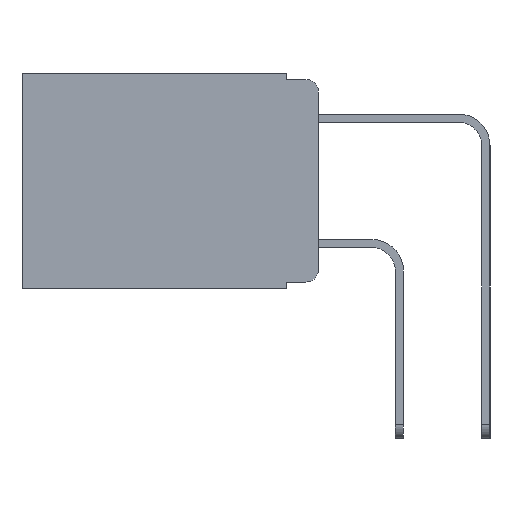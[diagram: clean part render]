
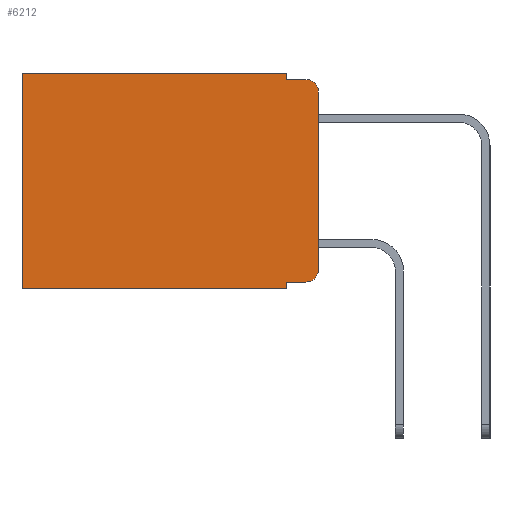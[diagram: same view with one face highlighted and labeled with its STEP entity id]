
A CAD part, left-side view. The second image highlights one B-rep face of the part: STEP entity #6212.
In plain terms, the highlighted planar face has unit normal (-1, 0, 0).
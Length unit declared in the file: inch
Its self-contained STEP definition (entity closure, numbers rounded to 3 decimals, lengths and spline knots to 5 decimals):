
#536 = LINE ( 'NONE', #10574, #8673 ) ;
#865 = CARTESIAN_POINT ( 'NONE',  ( 0.298, 0.473, 0. ) ) ;
#885 = ORIENTED_EDGE ( 'NONE', *, *, #20731, .F. ) ;
#1170 = ORIENTED_EDGE ( 'NONE', *, *, #5520, .T. ) ;
#1482 = VERTEX_POINT ( 'NONE', #12578 ) ;
#1558 = CIRCLE ( 'NONE', #4630, 0.02 ) ;
#2705 = EDGE_CURVE ( 'NONE', #1482, #16209, #9007, .T. ) ;
#2719 = ORIENTED_EDGE ( 'NONE', *, *, #12530, .T. ) ;
#3140 = CARTESIAN_POINT ( 'NONE',  ( 0.298, 0., -0.03 ) ) ;
#3523 = CARTESIAN_POINT ( 'NONE',  ( 0.298, 0., 0. ) ) ;
#3620 = CARTESIAN_POINT ( 'NONE',  ( 0.298, 0.02, -0.333 ) ) ;
#4028 = VECTOR ( 'NONE', #13603, 39.37008 ) ;
#4142 = VERTEX_POINT ( 'NONE', #865 ) ;
#4434 = CARTESIAN_POINT ( 'NONE',  ( 0.298, 0.02, -0.03 ) ) ;
#4630 = AXIS2_PLACEMENT_3D ( 'NONE', #4434, #22246, #15736 ) ;
#5473 = CARTESIAN_POINT ( 'NONE',  ( 0.298, 0., -0.313 ) ) ;
#5520 = EDGE_CURVE ( 'NONE', #17731, #4142, #17929, .T. ) ;
#5743 = CARTESIAN_POINT ( 'NONE',  ( 0.298, 0.051, -0.01 ) ) ;
#6090 = DIRECTION ( 'NONE',  ( 0., 0., -1. ) ) ;
#6212 = ADVANCED_FACE ( 'NONE', ( #18180 ), #18101, .F. ) ;
#6329 = DIRECTION ( 'NONE',  ( 0., 0., -1. ) ) ;
#6788 = VERTEX_POINT ( 'NONE', #5473 ) ;
#6921 = LINE ( 'NONE', #17741, #20232 ) ;
#7203 = VERTEX_POINT ( 'NONE', #14948 ) ;
#7598 = ORIENTED_EDGE ( 'NONE', *, *, #2705, .T. ) ;
#7611 = DIRECTION ( 'NONE',  ( 0., -1., 0. ) ) ;
#7871 = VERTEX_POINT ( 'NONE', #9380 ) ;
#8108 = CARTESIAN_POINT ( 'NONE',  ( 0.298, 0.473, -0.343 ) ) ;
#8127 = EDGE_CURVE ( 'NONE', #10082, #6788, #9394, .T. ) ;
#8179 = VECTOR ( 'NONE', #6090, 39.37008 ) ;
#8326 = ORIENTED_EDGE ( 'NONE', *, *, #8127, .F. ) ;
#8637 = VECTOR ( 'NONE', #7611, 39.37008 ) ;
#8649 = EDGE_CURVE ( 'NONE', #10082, #7871, #1558, .T. ) ;
#8673 = VECTOR ( 'NONE', #12392, 39.37008 ) ;
#8676 = EDGE_LOOP ( 'NONE', ( #8326, #15690, #21922, #22756, #1170, #11644, #885, #20040, #7598, #2719 ) ) ;
#8715 = DIRECTION ( 'NONE',  ( 0., 1., 0. ) ) ;
#9007 = LINE ( 'NONE', #18710, #22789 ) ;
#9380 = CARTESIAN_POINT ( 'NONE',  ( 0.298, 0.02, -0.01 ) ) ;
#9394 = LINE ( 'NONE', #3523, #13636 ) ;
#9458 = EDGE_CURVE ( 'NONE', #1482, #7203, #13002, .T. ) ;
#10082 = VERTEX_POINT ( 'NONE', #3140 ) ;
#10359 = VERTEX_POINT ( 'NONE', #11546 ) ;
#10502 = CARTESIAN_POINT ( 'NONE',  ( 0.298, 0.02, -0.313 ) ) ;
#10574 = CARTESIAN_POINT ( 'NONE',  ( 0.298, 0.473, 0. ) ) ;
#11546 = CARTESIAN_POINT ( 'NONE',  ( 0.298, 0.051, -0.01 ) ) ;
#11644 = ORIENTED_EDGE ( 'NONE', *, *, #20216, .T. ) ;
#11695 = CARTESIAN_POINT ( 'NONE',  ( 0.298, 0.051, 0. ) ) ;
#12268 = VECTOR ( 'NONE', #6329, 39.37008 ) ;
#12311 = DIRECTION ( 'NONE',  ( 0., 0., -1. ) ) ;
#12392 = DIRECTION ( 'NONE',  ( 0., 0., -1. ) ) ;
#12530 = EDGE_CURVE ( 'NONE', #16209, #6788, #13969, .T. ) ;
#12578 = CARTESIAN_POINT ( 'NONE',  ( 0.298, 0.051, -0.333 ) ) ;
#12847 = CARTESIAN_POINT ( 'NONE',  ( 0.298, 0., 0. ) ) ;
#13002 = LINE ( 'NONE', #22092, #8179 ) ;
#13455 = LINE ( 'NONE', #5743, #8637 ) ;
#13603 = DIRECTION ( 'NONE',  ( 0., 1., 0. ) ) ;
#13636 = VECTOR ( 'NONE', #17037, 39.37008 ) ;
#13969 = CIRCLE ( 'NONE', #21072, 0.02 ) ;
#14627 = EDGE_CURVE ( 'NONE', #10359, #7871, #13455, .T. ) ;
#14948 = CARTESIAN_POINT ( 'NONE',  ( 0.298, 0.051, -0.343 ) ) ;
#15690 = ORIENTED_EDGE ( 'NONE', *, *, #8649, .T. ) ;
#15736 = DIRECTION ( 'NONE',  ( 0., 0., -1. ) ) ;
#15979 = EDGE_CURVE ( 'NONE', #17731, #10359, #17637, .T. ) ;
#16209 = VERTEX_POINT ( 'NONE', #3620 ) ;
#16771 = AXIS2_PLACEMENT_3D ( 'NONE', #18052, #21897, #21844 ) ;
#17037 = DIRECTION ( 'NONE',  ( 0., 0., -1. ) ) ;
#17637 = LINE ( 'NONE', #18998, #12268 ) ;
#17731 = VERTEX_POINT ( 'NONE', #11695 ) ;
#17741 = CARTESIAN_POINT ( 'NONE',  ( 0.298, 0., -0.343 ) ) ;
#17929 = LINE ( 'NONE', #12847, #4028 ) ;
#18052 = CARTESIAN_POINT ( 'NONE',  ( 0.298, 0., 0. ) ) ;
#18101 = PLANE ( 'NONE',  #16771 ) ;
#18180 = FACE_OUTER_BOUND ( 'NONE', #8676, .T. ) ;
#18710 = CARTESIAN_POINT ( 'NONE',  ( 0.298, 0.051, -0.333 ) ) ;
#18998 = CARTESIAN_POINT ( 'NONE',  ( 0.298, 0.051, 0. ) ) ;
#19719 = DIRECTION ( 'NONE',  ( 0., -1., 0. ) ) ;
#20040 = ORIENTED_EDGE ( 'NONE', *, *, #9458, .F. ) ;
#20216 = EDGE_CURVE ( 'NONE', #4142, #22705, #536, .T. ) ;
#20232 = VECTOR ( 'NONE', #8715, 39.37008 ) ;
#20731 = EDGE_CURVE ( 'NONE', #7203, #22705, #6921, .T. ) ;
#21072 = AXIS2_PLACEMENT_3D ( 'NONE', #10502, #23029, #12311 ) ;
#21844 = DIRECTION ( 'NONE',  ( 0., 0., -1. ) ) ;
#21897 = DIRECTION ( 'NONE',  ( 1., 0., 0. ) ) ;
#21922 = ORIENTED_EDGE ( 'NONE', *, *, #14627, .F. ) ;
#22092 = CARTESIAN_POINT ( 'NONE',  ( 0.298, 0.051, 0. ) ) ;
#22246 = DIRECTION ( 'NONE',  ( -1., 0., 0. ) ) ;
#22705 = VERTEX_POINT ( 'NONE', #8108 ) ;
#22756 = ORIENTED_EDGE ( 'NONE', *, *, #15979, .F. ) ;
#22789 = VECTOR ( 'NONE', #19719, 39.37008 ) ;
#23029 = DIRECTION ( 'NONE',  ( -1., 0., 0. ) ) ;
